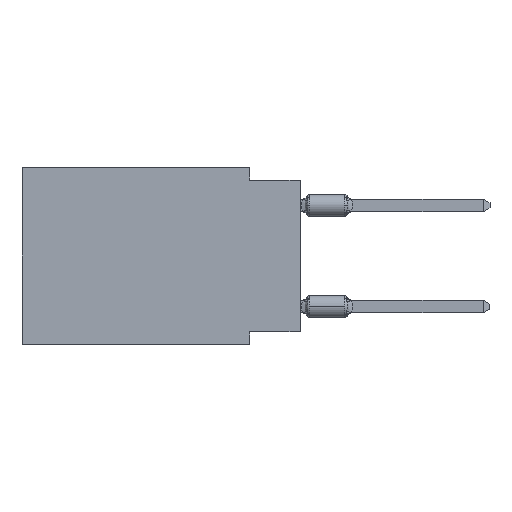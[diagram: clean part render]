
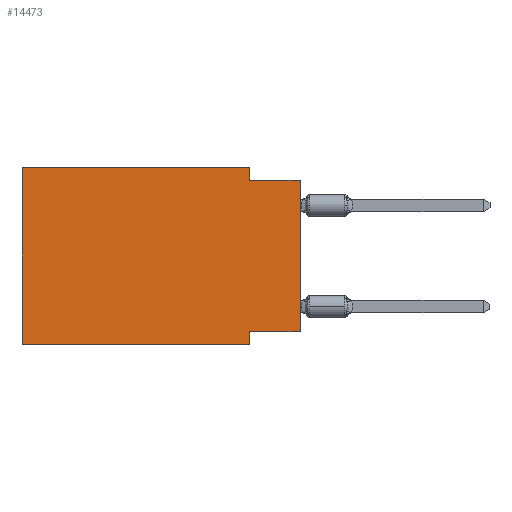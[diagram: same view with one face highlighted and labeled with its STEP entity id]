
A CAD part, left-side view. The second image highlights one B-rep face of the part: STEP entity #14473.
In plain terms, the highlighted planar face has unit normal (-1, 0, 0).
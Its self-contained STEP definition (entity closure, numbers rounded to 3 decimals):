
#82 = CARTESIAN_POINT ( 'NONE',  ( 0., 2.54, -8.89 ) ) ;
#92 = VERTEX_POINT ( 'NONE', #9357 ) ;
#150 = DIRECTION ( 'NONE',  ( 1., 0., 0. ) ) ;
#380 = ORIENTED_EDGE ( 'NONE', *, *, #11362, .F. ) ;
#992 = DIRECTION ( 'NONE',  ( 0., 0., 1. ) ) ;
#1301 = CARTESIAN_POINT ( 'NONE',  ( 0., 2.54, -8.89 ) ) ;
#1408 = PLANE ( 'NONE',  #11337 ) ;
#1527 = CARTESIAN_POINT ( 'NONE',  ( 0., 13.97, 0. ) ) ;
#1749 = CARTESIAN_POINT ( 'NONE',  ( 0., 0., 0. ) ) ;
#1898 = ORIENTED_EDGE ( 'NONE', *, *, #9162, .F. ) ;
#1958 = EDGE_CURVE ( 'NONE', #12067, #7299, #7166, .T. ) ;
#2715 = LINE ( 'NONE', #1301, #14056 ) ;
#2788 = EDGE_CURVE ( 'NONE', #6193, #14535, #3759, .T. ) ;
#2883 = VERTEX_POINT ( 'NONE', #14474 ) ;
#3194 = VECTOR ( 'NONE', #992, 1000. ) ;
#3249 = ORIENTED_EDGE ( 'NONE', *, *, #1958, .T. ) ;
#3378 = EDGE_CURVE ( 'NONE', #14535, #7299, #5915, .T. ) ;
#3759 = LINE ( 'NONE', #4930, #9096 ) ;
#3882 = VECTOR ( 'NONE', #10731, 1000. ) ;
#3908 = VECTOR ( 'NONE', #6561, 1000. ) ;
#4350 = DIRECTION ( 'NONE',  ( 0., 0., 1. ) ) ;
#4521 = DIRECTION ( 'NONE',  ( 0., 1., 0. ) ) ;
#4525 = CARTESIAN_POINT ( 'NONE',  ( 0., 0., -8.255 ) ) ;
#4598 = LINE ( 'NONE', #13474, #3882 ) ;
#4756 = ORIENTED_EDGE ( 'NONE', *, *, #12329, .F. ) ;
#4930 = CARTESIAN_POINT ( 'NONE',  ( 0., 2.54, 0. ) ) ;
#5020 = DIRECTION ( 'NONE',  ( 0., 0., -1. ) ) ;
#5518 = VECTOR ( 'NONE', #16135, 1000. ) ;
#5825 = CARTESIAN_POINT ( 'NONE',  ( 0., 13.97, 0. ) ) ;
#5915 = LINE ( 'NONE', #11018, #5518 ) ;
#6193 = VERTEX_POINT ( 'NONE', #13744 ) ;
#6561 = DIRECTION ( 'NONE',  ( 0., -1., 0. ) ) ;
#6743 = VECTOR ( 'NONE', #4350, 1000. ) ;
#7166 = LINE ( 'NONE', #1749, #3194 ) ;
#7299 = VERTEX_POINT ( 'NONE', #10581 ) ;
#7527 = ORIENTED_EDGE ( 'NONE', *, *, #10432, .F. ) ;
#7729 = CARTESIAN_POINT ( 'NONE',  ( 0., 13.97, -8.89 ) ) ;
#7762 = FACE_OUTER_BOUND ( 'NONE', #11565, .T. ) ;
#9096 = VECTOR ( 'NONE', #5020, 1000. ) ;
#9162 = EDGE_CURVE ( 'NONE', #11123, #6193, #4598, .T. ) ;
#9357 = CARTESIAN_POINT ( 'NONE',  ( 0., 13.97, -8.89 ) ) ;
#9486 = VERTEX_POINT ( 'NONE', #82 ) ;
#9812 = VECTOR ( 'NONE', #4521, 1000. ) ;
#10216 = EDGE_CURVE ( 'NONE', #92, #9486, #12679, .T. ) ;
#10432 = EDGE_CURVE ( 'NONE', #12067, #2883, #15927, .T. ) ;
#10490 = ORIENTED_EDGE ( 'NONE', *, *, #2788, .F. ) ;
#10581 = CARTESIAN_POINT ( 'NONE',  ( 0., 0., -0.635 ) ) ;
#10731 = DIRECTION ( 'NONE',  ( 0., -1., 0. ) ) ;
#10779 = CARTESIAN_POINT ( 'NONE',  ( 0., 2.54, -0.635 ) ) ;
#11018 = CARTESIAN_POINT ( 'NONE',  ( 0., 0., -0.635 ) ) ;
#11123 = VERTEX_POINT ( 'NONE', #5825 ) ;
#11337 = AXIS2_PLACEMENT_3D ( 'NONE', #11626, #150, #11714 ) ;
#11362 = EDGE_CURVE ( 'NONE', #2883, #9486, #2715, .T. ) ;
#11565 = EDGE_LOOP ( 'NONE', ( #3249, #16437, #10490, #1898, #4756, #15888, #380, #7527 ) ) ;
#11626 = CARTESIAN_POINT ( 'NONE',  ( 0., 13.97, 0. ) ) ;
#11714 = DIRECTION ( 'NONE',  ( 0., 0., -1. ) ) ;
#12067 = VERTEX_POINT ( 'NONE', #4525 ) ;
#12329 = EDGE_CURVE ( 'NONE', #92, #11123, #15845, .T. ) ;
#12679 = LINE ( 'NONE', #7729, #3908 ) ;
#12682 = DIRECTION ( 'NONE',  ( 0., 0., -1. ) ) ;
#13474 = CARTESIAN_POINT ( 'NONE',  ( 0., 13.97, 0. ) ) ;
#13744 = CARTESIAN_POINT ( 'NONE',  ( 0., 2.54, 0. ) ) ;
#14056 = VECTOR ( 'NONE', #12682, 1000. ) ;
#14473 = ADVANCED_FACE ( 'NONE', ( #7762 ), #1408, .F. ) ;
#14474 = CARTESIAN_POINT ( 'NONE',  ( 0., 2.54, -8.255 ) ) ;
#14535 = VERTEX_POINT ( 'NONE', #10779 ) ;
#14901 = CARTESIAN_POINT ( 'NONE',  ( 0., 0., -8.255 ) ) ;
#15845 = LINE ( 'NONE', #1527, #6743 ) ;
#15888 = ORIENTED_EDGE ( 'NONE', *, *, #10216, .T. ) ;
#15927 = LINE ( 'NONE', #14901, #9812 ) ;
#16135 = DIRECTION ( 'NONE',  ( 0., -1., 0. ) ) ;
#16437 = ORIENTED_EDGE ( 'NONE', *, *, #3378, .F. ) ;
